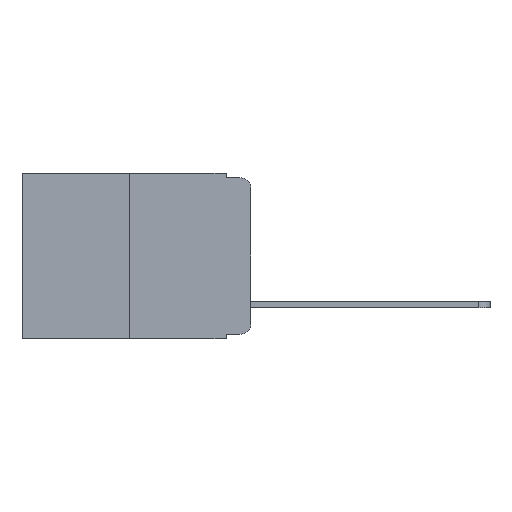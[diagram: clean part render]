
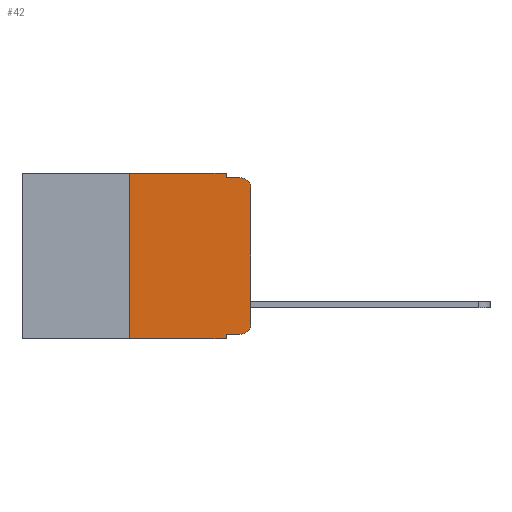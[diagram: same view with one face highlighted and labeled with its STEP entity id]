
A CAD part, left-side view. The second image highlights one B-rep face of the part: STEP entity #42.
In plain terms, the highlighted planar face has unit normal (-1, 0, 0).
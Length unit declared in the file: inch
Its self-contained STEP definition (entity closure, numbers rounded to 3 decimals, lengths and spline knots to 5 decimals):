
#27 = CARTESIAN_POINT ( 'NONE',  ( 0., 0.473, -0.343 ) ) ;
#42 = ADVANCED_FACE ( 'NONE', ( #12769 ), #11709, .F. ) ;
#504 = VECTOR ( 'NONE', #19234, 39.37008 ) ;
#538 = ORIENTED_EDGE ( 'NONE', *, *, #3710, .T. ) ;
#1459 = VERTEX_POINT ( 'NONE', #4876 ) ;
#1930 = ORIENTED_EDGE ( 'NONE', *, *, #7474, .T. ) ;
#1972 = CARTESIAN_POINT ( 'NONE',  ( 0., 0.051, -0.01 ) ) ;
#2001 = EDGE_CURVE ( 'NONE', #8992, #9044, #16821, .T. ) ;
#2522 = VECTOR ( 'NONE', #11802, 39.37008 ) ;
#3255 = VERTEX_POINT ( 'NONE', #6388 ) ;
#3375 = VERTEX_POINT ( 'NONE', #17911 ) ;
#3413 = VERTEX_POINT ( 'NONE', #15337 ) ;
#3710 = EDGE_CURVE ( 'NONE', #3413, #11877, #14929, .T. ) ;
#4426 = VECTOR ( 'NONE', #15817, 39.37008 ) ;
#4528 = EDGE_CURVE ( 'NONE', #3413, #3375, #19001, .T. ) ;
#4607 = CARTESIAN_POINT ( 'NONE',  ( 0., 0.02, -0.01 ) ) ;
#4876 = CARTESIAN_POINT ( 'NONE',  ( 0., 0.051, 0. ) ) ;
#5558 = AXIS2_PLACEMENT_3D ( 'NONE', #16638, #8034, #17841 ) ;
#5892 = VECTOR ( 'NONE', #13657, 39.37008 ) ;
#5926 = DIRECTION ( 'NONE',  ( 0., 0., -1. ) ) ;
#6169 = AXIS2_PLACEMENT_3D ( 'NONE', #7977, #9200, #11703 ) ;
#6388 = CARTESIAN_POINT ( 'NONE',  ( 0., 0.051, -0.01 ) ) ;
#6413 = LINE ( 'NONE', #17621, #13759 ) ;
#6565 = CARTESIAN_POINT ( 'NONE',  ( 0., 0.051, 0. ) ) ;
#6877 = VECTOR ( 'NONE', #7674, 39.37008 ) ;
#6989 = ORIENTED_EDGE ( 'NONE', *, *, #19569, .F. ) ;
#7335 = EDGE_CURVE ( 'NONE', #8992, #3375, #17928, .T. ) ;
#7474 = EDGE_CURVE ( 'NONE', #11877, #15285, #12467, .T. ) ;
#7674 = DIRECTION ( 'NONE',  ( 0., 0., -1. ) ) ;
#7977 = CARTESIAN_POINT ( 'NONE',  ( 0., 0.473, 0. ) ) ;
#8034 = DIRECTION ( 'NONE',  ( -1., 0., 0. ) ) ;
#8045 = ORIENTED_EDGE ( 'NONE', *, *, #14837, .T. ) ;
#8272 = CARTESIAN_POINT ( 'NONE',  ( 0., 0., 0. ) ) ;
#8494 = ORIENTED_EDGE ( 'NONE', *, *, #4528, .F. ) ;
#8713 = CARTESIAN_POINT ( 'NONE',  ( 0., 0.473, 0. ) ) ;
#8810 = ORIENTED_EDGE ( 'NONE', *, *, #14099, .T. ) ;
#8992 = VERTEX_POINT ( 'NONE', #12040 ) ;
#9044 = VERTEX_POINT ( 'NONE', #18620 ) ;
#9200 = DIRECTION ( 'NONE',  ( 1., 0., 0. ) ) ;
#9396 = LINE ( 'NONE', #1972, #12928 ) ;
#9553 = EDGE_LOOP ( 'NONE', ( #8810, #8045, #16391, #6989, #13561, #15606, #14488, #8494, #538, #1930 ) ) ;
#10349 = CARTESIAN_POINT ( 'NONE',  ( 0., 0., -0.313 ) ) ;
#10357 = CIRCLE ( 'NONE', #5558, 0.02 ) ;
#10391 = DIRECTION ( 'NONE',  ( -1., 0., 0. ) ) ;
#11703 = DIRECTION ( 'NONE',  ( 0., 0., -1. ) ) ;
#11709 = PLANE ( 'NONE',  #6169 ) ;
#11750 = CARTESIAN_POINT ( 'NONE',  ( 0., 0.051, -0.333 ) ) ;
#11802 = DIRECTION ( 'NONE',  ( 0., -1., 0. ) ) ;
#11877 = VERTEX_POINT ( 'NONE', #18284 ) ;
#12040 = CARTESIAN_POINT ( 'NONE',  ( 0., 0.25, -0.343 ) ) ;
#12467 = CIRCLE ( 'NONE', #16187, 0.02 ) ;
#12769 = FACE_OUTER_BOUND ( 'NONE', #9553, .T. ) ;
#12928 = VECTOR ( 'NONE', #18682, 39.37008 ) ;
#13169 = LINE ( 'NONE', #8713, #4426 ) ;
#13364 = VECTOR ( 'NONE', #17592, 39.37008 ) ;
#13536 = LINE ( 'NONE', #8272, #504 ) ;
#13561 = ORIENTED_EDGE ( 'NONE', *, *, #16814, .F. ) ;
#13657 = DIRECTION ( 'NONE',  ( 0., -1., 0. ) ) ;
#13759 = VECTOR ( 'NONE', #5926, 39.37008 ) ;
#14099 = EDGE_CURVE ( 'NONE', #15285, #15003, #13536, .T. ) ;
#14488 = ORIENTED_EDGE ( 'NONE', *, *, #7335, .T. ) ;
#14837 = EDGE_CURVE ( 'NONE', #15003, #14937, #10357, .T. ) ;
#14929 = LINE ( 'NONE', #11750, #2522 ) ;
#14937 = VERTEX_POINT ( 'NONE', #4607 ) ;
#15003 = VERTEX_POINT ( 'NONE', #19263 ) ;
#15285 = VERTEX_POINT ( 'NONE', #10349 ) ;
#15337 = CARTESIAN_POINT ( 'NONE',  ( 0., 0.051, -0.333 ) ) ;
#15606 = ORIENTED_EDGE ( 'NONE', *, *, #2001, .F. ) ;
#15817 = DIRECTION ( 'NONE',  ( 0., -1., 0. ) ) ;
#16187 = AXIS2_PLACEMENT_3D ( 'NONE', #18350, #10391, #19563 ) ;
#16391 = ORIENTED_EDGE ( 'NONE', *, *, #18417, .F. ) ;
#16638 = CARTESIAN_POINT ( 'NONE',  ( 0., 0.02, -0.03 ) ) ;
#16814 = EDGE_CURVE ( 'NONE', #9044, #1459, #13169, .T. ) ;
#16821 = LINE ( 'NONE', #17283, #13364 ) ;
#17283 = CARTESIAN_POINT ( 'NONE',  ( 0., 0.25, 0. ) ) ;
#17592 = DIRECTION ( 'NONE',  ( 0., 0., 1. ) ) ;
#17621 = CARTESIAN_POINT ( 'NONE',  ( 0., 0.051, 0. ) ) ;
#17841 = DIRECTION ( 'NONE',  ( 0., 0., -1. ) ) ;
#17911 = CARTESIAN_POINT ( 'NONE',  ( 0., 0.051, -0.343 ) ) ;
#17928 = LINE ( 'NONE', #27, #5892 ) ;
#18284 = CARTESIAN_POINT ( 'NONE',  ( 0., 0.02, -0.333 ) ) ;
#18350 = CARTESIAN_POINT ( 'NONE',  ( 0., 0.02, -0.313 ) ) ;
#18417 = EDGE_CURVE ( 'NONE', #3255, #14937, #9396, .T. ) ;
#18620 = CARTESIAN_POINT ( 'NONE',  ( 0., 0.25, 0. ) ) ;
#18682 = DIRECTION ( 'NONE',  ( 0., -1., 0. ) ) ;
#19001 = LINE ( 'NONE', #6565, #6877 ) ;
#19234 = DIRECTION ( 'NONE',  ( 0., 0., 1. ) ) ;
#19263 = CARTESIAN_POINT ( 'NONE',  ( 0., 0., -0.03 ) ) ;
#19563 = DIRECTION ( 'NONE',  ( 0., 0., -1. ) ) ;
#19569 = EDGE_CURVE ( 'NONE', #1459, #3255, #6413, .T. ) ;
